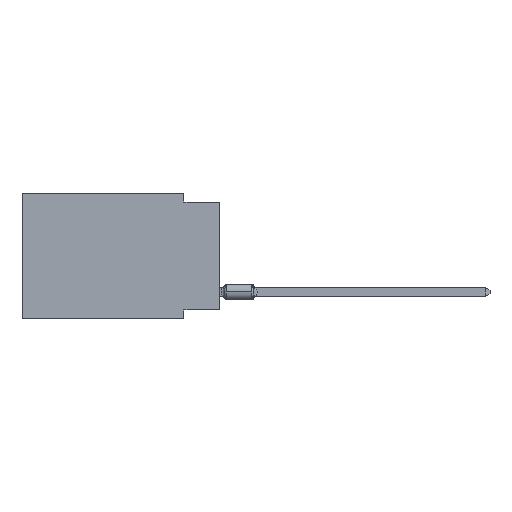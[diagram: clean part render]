
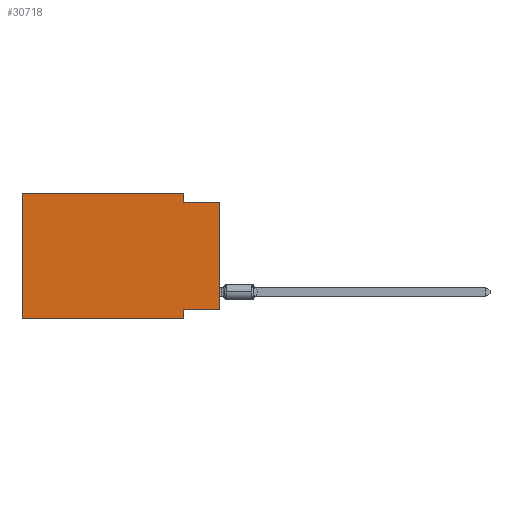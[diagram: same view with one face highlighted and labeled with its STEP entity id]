
A CAD part, left-side view. The second image highlights one B-rep face of the part: STEP entity #30718.
In plain terms, the highlighted planar face has unit normal (-1, 0, 0).
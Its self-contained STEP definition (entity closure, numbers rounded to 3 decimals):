
#905 = DIRECTION ( 'NONE',  ( 0., 0., -1. ) ) ;
#1886 = CARTESIAN_POINT ( 'NONE',  ( 0., 0., -0.635 ) ) ;
#4718 = CARTESIAN_POINT ( 'NONE',  ( 0., 2.54, 0. ) ) ;
#4731 = VECTOR ( 'NONE', #13215, 1000. ) ;
#4888 = VECTOR ( 'NONE', #13995, 1000. ) ;
#5187 = VERTEX_POINT ( 'NONE', #25638 ) ;
#5285 = VECTOR ( 'NONE', #18194, 1000. ) ;
#6130 = DIRECTION ( 'NONE',  ( 0., 0., 1. ) ) ;
#6149 = ORIENTED_EDGE ( 'NONE', *, *, #6869, .F. ) ;
#6869 = EDGE_CURVE ( 'NONE', #10744, #33132, #18710, .T. ) ;
#7431 = DIRECTION ( 'NONE',  ( 0., -1., 0. ) ) ;
#8892 = EDGE_CURVE ( 'NONE', #33132, #14621, #27854, .T. ) ;
#10124 = CARTESIAN_POINT ( 'NONE',  ( 0., 13.97, 0. ) ) ;
#10744 = VERTEX_POINT ( 'NONE', #30731 ) ;
#11773 = ORIENTED_EDGE ( 'NONE', *, *, #14702, .T. ) ;
#12066 = DIRECTION ( 'NONE',  ( 0., 0., -1. ) ) ;
#12163 = CARTESIAN_POINT ( 'NONE',  ( 0., 2.54, -0.635 ) ) ;
#13215 = DIRECTION ( 'NONE',  ( 0., -1., 0. ) ) ;
#13450 = ORIENTED_EDGE ( 'NONE', *, *, #8892, .F. ) ;
#13815 = VERTEX_POINT ( 'NONE', #20792 ) ;
#13995 = DIRECTION ( 'NONE',  ( 0., 0., -1. ) ) ;
#14166 = EDGE_LOOP ( 'NONE', ( #11773, #30546, #17025, #13450, #6149, #27622, #32120, #18779 ) ) ;
#14621 = VERTEX_POINT ( 'NONE', #4718 ) ;
#14702 = EDGE_CURVE ( 'NONE', #35686, #13815, #27263, .T. ) ;
#15542 = CARTESIAN_POINT ( 'NONE',  ( 0., 2.54, -8.89 ) ) ;
#17025 = ORIENTED_EDGE ( 'NONE', *, *, #23914, .F. ) ;
#17069 = LINE ( 'NONE', #1886, #38833 ) ;
#17666 = CARTESIAN_POINT ( 'NONE',  ( 0., 2.54, 0. ) ) ;
#18194 = DIRECTION ( 'NONE',  ( 0., -1., 0. ) ) ;
#18501 = CARTESIAN_POINT ( 'NONE',  ( 0., 0., -8.255 ) ) ;
#18606 = VERTEX_POINT ( 'NONE', #12163 ) ;
#18710 = LINE ( 'NONE', #31032, #26134 ) ;
#18779 = ORIENTED_EDGE ( 'NONE', *, *, #32133, .F. ) ;
#19316 = LINE ( 'NONE', #18501, #32257 ) ;
#19321 = DIRECTION ( 'NONE',  ( 0., 0., 1. ) ) ;
#19611 = VERTEX_POINT ( 'NONE', #31140 ) ;
#19972 = CARTESIAN_POINT ( 'NONE',  ( 0., 13.97, -8.89 ) ) ;
#19988 = EDGE_CURVE ( 'NONE', #18606, #13815, #17069, .T. ) ;
#20792 = CARTESIAN_POINT ( 'NONE',  ( 0., 0., -0.635 ) ) ;
#20920 = PLANE ( 'NONE',  #26148 ) ;
#22667 = CARTESIAN_POINT ( 'NONE',  ( 0., 0., -8.255 ) ) ;
#23914 = EDGE_CURVE ( 'NONE', #14621, #18606, #39210, .T. ) ;
#24580 = CARTESIAN_POINT ( 'NONE',  ( 0., 0., 0. ) ) ;
#25638 = CARTESIAN_POINT ( 'NONE',  ( 0., 2.54, -8.255 ) ) ;
#25782 = VECTOR ( 'NONE', #12066, 1000. ) ;
#26134 = VECTOR ( 'NONE', #19321, 1000. ) ;
#26148 = AXIS2_PLACEMENT_3D ( 'NONE', #10124, #29385, #905 ) ;
#27263 = LINE ( 'NONE', #24580, #39189 ) ;
#27622 = ORIENTED_EDGE ( 'NONE', *, *, #38204, .T. ) ;
#27854 = LINE ( 'NONE', #40353, #5285 ) ;
#28561 = CARTESIAN_POINT ( 'NONE',  ( 0., 13.97, 0. ) ) ;
#29385 = DIRECTION ( 'NONE',  ( 1., 0., 0. ) ) ;
#30546 = ORIENTED_EDGE ( 'NONE', *, *, #19988, .F. ) ;
#30718 = ADVANCED_FACE ( 'NONE', ( #38228 ), #20920, .F. ) ;
#30731 = CARTESIAN_POINT ( 'NONE',  ( 0., 13.97, -8.89 ) ) ;
#31032 = CARTESIAN_POINT ( 'NONE',  ( 0., 13.97, 0. ) ) ;
#31140 = CARTESIAN_POINT ( 'NONE',  ( 0., 2.54, -8.89 ) ) ;
#32120 = ORIENTED_EDGE ( 'NONE', *, *, #35127, .F. ) ;
#32133 = EDGE_CURVE ( 'NONE', #35686, #5187, #19316, .T. ) ;
#32257 = VECTOR ( 'NONE', #37980, 1000. ) ;
#33132 = VERTEX_POINT ( 'NONE', #28561 ) ;
#35127 = EDGE_CURVE ( 'NONE', #5187, #19611, #40171, .T. ) ;
#35138 = LINE ( 'NONE', #19972, #4731 ) ;
#35686 = VERTEX_POINT ( 'NONE', #22667 ) ;
#37980 = DIRECTION ( 'NONE',  ( 0., 1., 0. ) ) ;
#38204 = EDGE_CURVE ( 'NONE', #10744, #19611, #35138, .T. ) ;
#38228 = FACE_OUTER_BOUND ( 'NONE', #14166, .T. ) ;
#38833 = VECTOR ( 'NONE', #7431, 1000. ) ;
#39189 = VECTOR ( 'NONE', #6130, 1000. ) ;
#39210 = LINE ( 'NONE', #17666, #4888 ) ;
#40171 = LINE ( 'NONE', #15542, #25782 ) ;
#40353 = CARTESIAN_POINT ( 'NONE',  ( 0., 13.97, 0. ) ) ;
